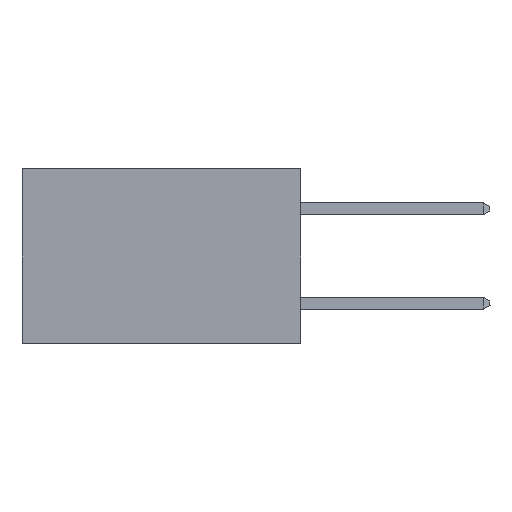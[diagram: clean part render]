
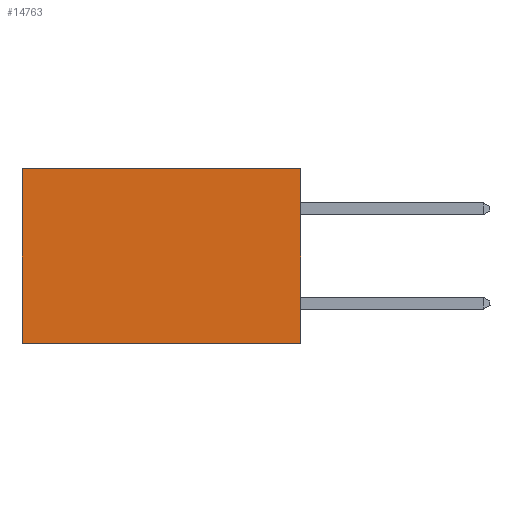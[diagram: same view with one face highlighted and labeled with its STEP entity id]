
A CAD part, left-side view. The second image highlights one B-rep face of the part: STEP entity #14763.
In plain terms, the highlighted planar face has unit normal (-1, 0, 0).
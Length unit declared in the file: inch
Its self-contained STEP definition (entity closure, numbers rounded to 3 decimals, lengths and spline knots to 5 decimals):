
#955 = DIRECTION ( 'NONE',  ( 0., 0., -1. ) ) ;
#1026 = VERTEX_POINT ( 'NONE', #18048 ) ;
#1801 = DIRECTION ( 'NONE',  ( 0., 0., -1. ) ) ;
#1808 = VERTEX_POINT ( 'NONE', #24752 ) ;
#2403 = VECTOR ( 'NONE', #955, 39.37008 ) ;
#2445 = EDGE_LOOP ( 'NONE', ( #16826, #23437, #3136, #23050 ) ) ;
#3136 = ORIENTED_EDGE ( 'NONE', *, *, #13496, .F. ) ;
#4020 = LINE ( 'NONE', #10641, #25584 ) ;
#4834 = DIRECTION ( 'NONE',  ( 0., 1., 0. ) ) ;
#4851 = FACE_OUTER_BOUND ( 'NONE', #2445, .T. ) ;
#7868 = EDGE_CURVE ( 'NONE', #1808, #8521, #14719, .T. ) ;
#8062 = LINE ( 'NONE', #22476, #23122 ) ;
#8521 = VERTEX_POINT ( 'NONE', #10172 ) ;
#10172 = CARTESIAN_POINT ( 'NONE',  ( 0.277, 0.59, 0. ) ) ;
#10641 = CARTESIAN_POINT ( 'NONE',  ( 0.277, 0.59, -0.37 ) ) ;
#11735 = CARTESIAN_POINT ( 'NONE',  ( 0.277, 0., -0.37 ) ) ;
#13496 = EDGE_CURVE ( 'NONE', #1808, #23188, #23388, .T. ) ;
#13708 = DIRECTION ( 'NONE',  ( 1., 0., 0. ) ) ;
#14719 = LINE ( 'NONE', #18067, #19955 ) ;
#14763 = ADVANCED_FACE ( 'NONE', ( #4851 ), #23487, .F. ) ;
#16826 = ORIENTED_EDGE ( 'NONE', *, *, #24385, .T. ) ;
#17658 = DIRECTION ( 'NONE',  ( 0., 1., 0. ) ) ;
#18048 = CARTESIAN_POINT ( 'NONE',  ( 0.277, 0.59, -0.37 ) ) ;
#18067 = CARTESIAN_POINT ( 'NONE',  ( 0.277, 0., 0. ) ) ;
#19955 = VECTOR ( 'NONE', #17658, 39.37008 ) ;
#21775 = AXIS2_PLACEMENT_3D ( 'NONE', #11735, #13708, #1801 ) ;
#22476 = CARTESIAN_POINT ( 'NONE',  ( 0.277, 0., -0.37 ) ) ;
#22523 = CARTESIAN_POINT ( 'NONE',  ( 0.277, 0., -0.37 ) ) ;
#23050 = ORIENTED_EDGE ( 'NONE', *, *, #7868, .T. ) ;
#23122 = VECTOR ( 'NONE', #4834, 39.37008 ) ;
#23188 = VERTEX_POINT ( 'NONE', #22523 ) ;
#23388 = LINE ( 'NONE', #24664, #2403 ) ;
#23437 = ORIENTED_EDGE ( 'NONE', *, *, #24432, .F. ) ;
#23487 = PLANE ( 'NONE',  #21775 ) ;
#24359 = DIRECTION ( 'NONE',  ( 0., 0., -1. ) ) ;
#24385 = EDGE_CURVE ( 'NONE', #8521, #1026, #4020, .T. ) ;
#24432 = EDGE_CURVE ( 'NONE', #23188, #1026, #8062, .T. ) ;
#24664 = CARTESIAN_POINT ( 'NONE',  ( 0.277, 0., -0.37 ) ) ;
#24752 = CARTESIAN_POINT ( 'NONE',  ( 0.277, 0., 0. ) ) ;
#25584 = VECTOR ( 'NONE', #24359, 39.37008 ) ;
